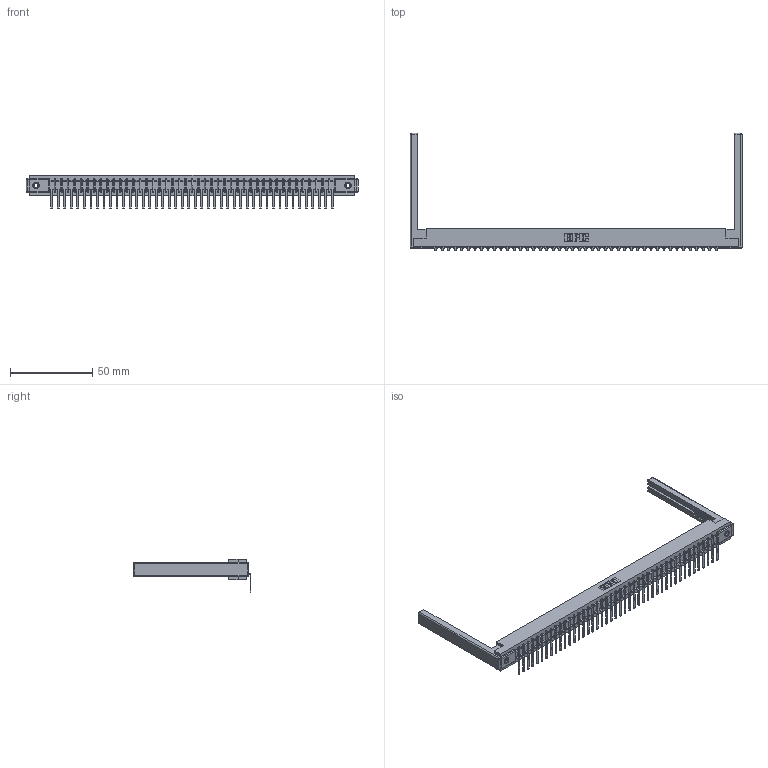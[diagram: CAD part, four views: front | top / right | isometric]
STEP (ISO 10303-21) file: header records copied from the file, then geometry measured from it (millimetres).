
FILE_DESCRIPTION (( 'STEP AP203' ), '1' );
FILE_NAME ('307-044-457-168.STEP', '2020-09-29T23:28:35', ( '' ), ( '' ), 'SwSTEP 2.0', 'SolidWorks 2020', '' );
FILE_SCHEMA (( 'CONFIG_CONTROL_DESIGN' ));
Length unit declared in the file: inch
Products named in the file (5): 307-044-457-168; 307-290-002_557; 345-250-001_345-250-001-102; 307-220-068; 307 Part_.156 Dia Mounting Holes
Assembly tree (49 placements, depth 2):
  307-044-457-168
    307 Part_.156 Dia Mounting Holes
    307-290-002_557  x44
    307-220-068  x2
    345-250-001_345-250-001-102  x2
Bounding box: 201.78 x 71.29 x 20.66 mm (x, y, z)
Volume: 26104 mm3; surface area: 32094.4 mm2
Topology: 49 solids, 49 shells, 3749 faces, 11449 edges, 7490 vertices
Faces by surface type: plane 2226, cylinder 1409, sphere 98, cone 12, torus 4
Entity records: 41087 total; most frequent: CARTESIAN_POINT 6897, ORIENTED_EDGE 6876, DIRECTION 6718, EDGE_CURVE 3438, LINE 2632, VECTOR 2632, VERTEX_POINT 2222, AXIS2_PLACEMENT_3D 2043
